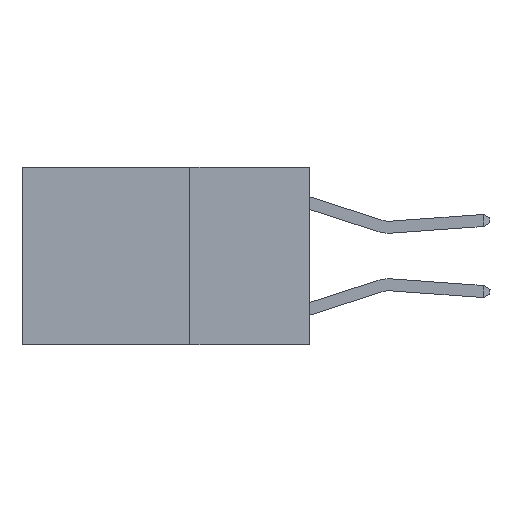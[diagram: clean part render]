
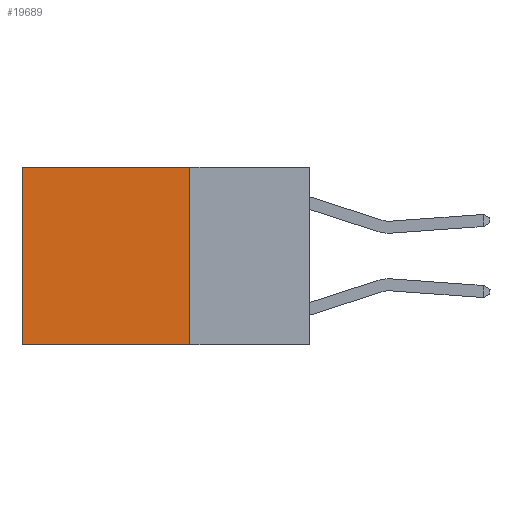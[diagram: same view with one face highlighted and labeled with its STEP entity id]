
A CAD part, left-side view. The second image highlights one B-rep face of the part: STEP entity #19689.
In plain terms, the highlighted planar face has unit normal (-1, 0, 0).
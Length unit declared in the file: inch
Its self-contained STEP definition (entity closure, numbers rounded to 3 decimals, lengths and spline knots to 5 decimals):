
#639 = AXIS2_PLACEMENT_3D ( 'NONE', #12608, #14772, #1719 ) ;
#855 = VERTEX_POINT ( 'NONE', #18687 ) ;
#1477 = CARTESIAN_POINT ( 'NONE',  ( 0.2625, 0.6, 0. ) ) ;
#1719 = DIRECTION ( 'NONE',  ( 0., 0., -1. ) ) ;
#1728 = EDGE_CURVE ( 'NONE', #20339, #855, #11080, .T. ) ;
#3681 = DIRECTION ( 'NONE',  ( 0., 0., -1. ) ) ;
#4285 = CARTESIAN_POINT ( 'NONE',  ( 0.2625, 0.25, 0. ) ) ;
#5252 = VECTOR ( 'NONE', #7038, 39.37008 ) ;
#6276 = CARTESIAN_POINT ( 'NONE',  ( 0.2625, 0.25, 0. ) ) ;
#7038 = DIRECTION ( 'NONE',  ( 0., 1., 0. ) ) ;
#7902 = EDGE_CURVE ( 'NONE', #20339, #15709, #13927, .T. ) ;
#11080 = LINE ( 'NONE', #26937, #5252 ) ;
#11089 = VERTEX_POINT ( 'NONE', #15990 ) ;
#11471 = DIRECTION ( 'NONE',  ( 0., 1., 0. ) ) ;
#12168 = LINE ( 'NONE', #1477, #23010 ) ;
#12608 = CARTESIAN_POINT ( 'NONE',  ( 0.2625, 0.25, 0. ) ) ;
#12887 = EDGE_CURVE ( 'NONE', #15709, #11089, #19168, .T. ) ;
#13298 = ORIENTED_EDGE ( 'NONE', *, *, #12887, .F. ) ;
#13927 = LINE ( 'NONE', #4285, #24723 ) ;
#14772 = DIRECTION ( 'NONE',  ( 1., 0., 0. ) ) ;
#15424 = EDGE_LOOP ( 'NONE', ( #21913, #13298, #23671, #27353 ) ) ;
#15709 = VERTEX_POINT ( 'NONE', #22933 ) ;
#15990 = CARTESIAN_POINT ( 'NONE',  ( 0.2625, 0.6, -0.37 ) ) ;
#17408 = DIRECTION ( 'NONE',  ( 0., 0., -1. ) ) ;
#17602 = EDGE_CURVE ( 'NONE', #855, #11089, #12168, .T. ) ;
#18687 = CARTESIAN_POINT ( 'NONE',  ( 0.2625, 0.6, 0. ) ) ;
#19168 = LINE ( 'NONE', #24412, #24885 ) ;
#19689 = ADVANCED_FACE ( 'NONE', ( #22338 ), #25527, .F. ) ;
#20339 = VERTEX_POINT ( 'NONE', #6276 ) ;
#21913 = ORIENTED_EDGE ( 'NONE', *, *, #17602, .T. ) ;
#22338 = FACE_OUTER_BOUND ( 'NONE', #15424, .T. ) ;
#22933 = CARTESIAN_POINT ( 'NONE',  ( 0.2625, 0.25, -0.37 ) ) ;
#23010 = VECTOR ( 'NONE', #3681, 39.37008 ) ;
#23671 = ORIENTED_EDGE ( 'NONE', *, *, #7902, .F. ) ;
#24412 = CARTESIAN_POINT ( 'NONE',  ( 0.2625, 0.25, -0.37 ) ) ;
#24723 = VECTOR ( 'NONE', #17408, 39.37008 ) ;
#24885 = VECTOR ( 'NONE', #11471, 39.37008 ) ;
#25527 = PLANE ( 'NONE',  #639 ) ;
#26937 = CARTESIAN_POINT ( 'NONE',  ( 0.2625, 0.25, 0. ) ) ;
#27353 = ORIENTED_EDGE ( 'NONE', *, *, #1728, .T. ) ;
